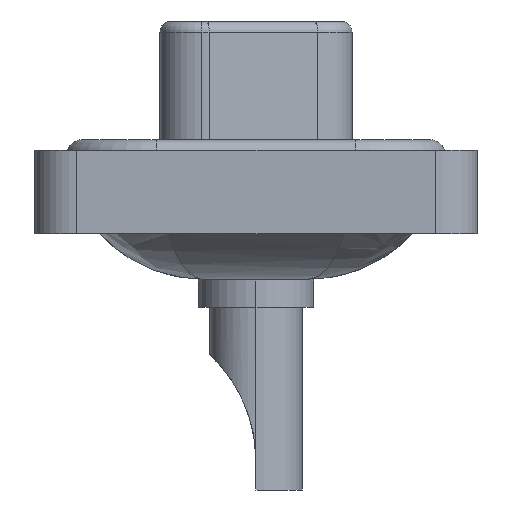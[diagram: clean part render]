
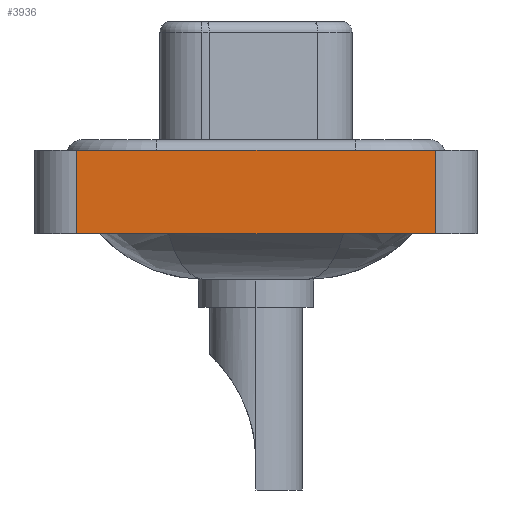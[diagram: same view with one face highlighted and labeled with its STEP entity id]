
A CAD part, left-side view. The second image highlights one B-rep face of the part: STEP entity #3936.
In plain terms, the highlighted planar face has unit normal (-1, 0, 0).
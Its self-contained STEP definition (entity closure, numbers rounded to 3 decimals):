
#815 = CARTESIAN_POINT ( 'NONE',  ( -7.35, 8.55, 0.4 ) ) ;
#826 = CARTESIAN_POINT ( 'NONE',  ( -7.35, -8.55, 0.4 ) ) ;
#990 = LINE ( 'NONE', #20145, #5462 ) ;
#1148 = DIRECTION ( 'NONE',  ( 0., 0., 1. ) ) ;
#1159 = VERTEX_POINT ( 'NONE', #7969 ) ;
#1202 = DIRECTION ( 'NONE',  ( 0., -1., 0. ) ) ;
#1344 = VERTEX_POINT ( 'NONE', #826 ) ;
#2607 = AXIS2_PLACEMENT_3D ( 'NONE', #4772, #14261, #1148 ) ;
#3936 = ADVANCED_FACE ( 'NONE', ( #19142 ), #17340, .T. ) ;
#4230 = CARTESIAN_POINT ( 'NONE',  ( -7.35, -8.55, 0.4 ) ) ;
#4772 = CARTESIAN_POINT ( 'NONE',  ( -7.35, -8.55, -3.6 ) ) ;
#5174 = ORIENTED_EDGE ( 'NONE', *, *, #15649, .F. ) ;
#5462 = VECTOR ( 'NONE', #12393, 1000. ) ;
#7532 = LINE ( 'NONE', #4230, #18196 ) ;
#7969 = CARTESIAN_POINT ( 'NONE',  ( -7.35, 8.55, -3.6 ) ) ;
#8083 = EDGE_CURVE ( 'NONE', #1159, #15073, #15679, .T. ) ;
#8430 = DIRECTION ( 'NONE',  ( 0., 0., 1. ) ) ;
#10362 = ORIENTED_EDGE ( 'NONE', *, *, #13282, .F. ) ;
#10801 = ORIENTED_EDGE ( 'NONE', *, *, #8083, .T. ) ;
#10841 = VECTOR ( 'NONE', #8430, 1000. ) ;
#11735 = CARTESIAN_POINT ( 'NONE',  ( -7.35, -8.55, -3.6 ) ) ;
#11848 = LINE ( 'NONE', #11735, #10841 ) ;
#12341 = DIRECTION ( 'NONE',  ( 0., -1., 0. ) ) ;
#12393 = DIRECTION ( 'NONE',  ( 0., 0., 1. ) ) ;
#12407 = CARTESIAN_POINT ( 'NONE',  ( -7.35, -8.55, -3.6 ) ) ;
#13282 = EDGE_CURVE ( 'NONE', #19618, #1344, #7532, .T. ) ;
#14261 = DIRECTION ( 'NONE',  ( -1., 0., 0. ) ) ;
#14411 = EDGE_LOOP ( 'NONE', ( #19742, #10362, #5174, #10801 ) ) ;
#14689 = VECTOR ( 'NONE', #1202, 1000. ) ;
#15073 = VERTEX_POINT ( 'NONE', #20590 ) ;
#15649 = EDGE_CURVE ( 'NONE', #1159, #19618, #990, .T. ) ;
#15679 = LINE ( 'NONE', #12407, #14689 ) ;
#17159 = EDGE_CURVE ( 'NONE', #15073, #1344, #11848, .T. ) ;
#17340 = PLANE ( 'NONE',  #2607 ) ;
#18196 = VECTOR ( 'NONE', #12341, 1000. ) ;
#19142 = FACE_OUTER_BOUND ( 'NONE', #14411, .T. ) ;
#19618 = VERTEX_POINT ( 'NONE', #815 ) ;
#19742 = ORIENTED_EDGE ( 'NONE', *, *, #17159, .T. ) ;
#20145 = CARTESIAN_POINT ( 'NONE',  ( -7.35, 8.55, -3.6 ) ) ;
#20590 = CARTESIAN_POINT ( 'NONE',  ( -7.35, -8.55, -3.6 ) ) ;
